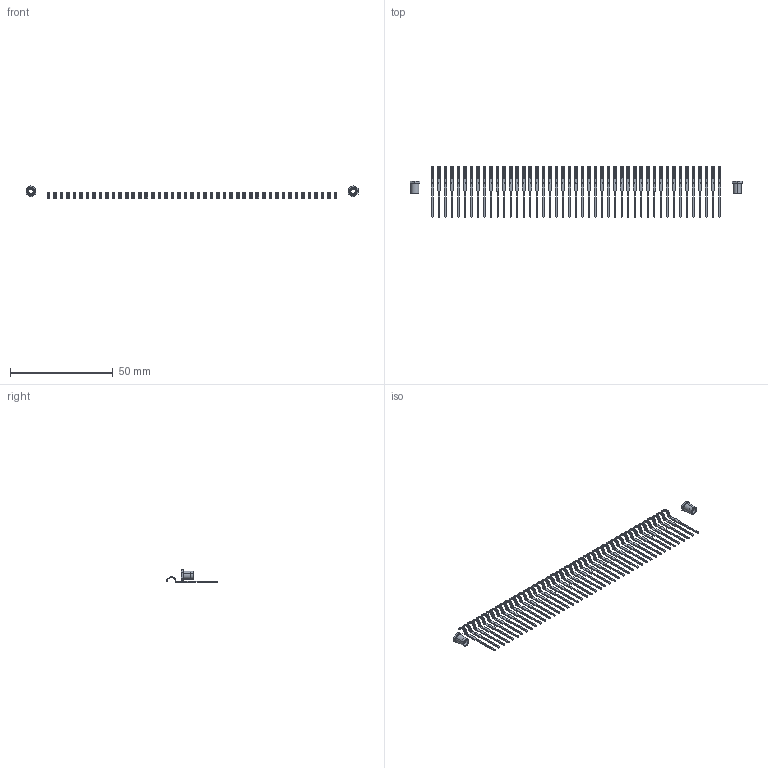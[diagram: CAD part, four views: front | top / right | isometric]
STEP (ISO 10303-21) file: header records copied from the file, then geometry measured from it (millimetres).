
FILE_DESCRIPTION (( 'STEP AP203' ), '1' );
FILE_NAME ('346-045-522-108.STEP', '2018-08-25T03:36:34', ( '' ), ( '' ), 'SwSTEP 2.0', 'SolidWorks 2016', '' );
FILE_SCHEMA (( 'CONFIG_CONTROL_DESIGN' ));
Length unit declared in the file: inch
Products named in the file (4): 345-250-001_345-250-003-102; 346-045-522-108; 346 Part_Flush Mounting Lugs - 0.156 Dia-TI; 345-292-001_345-293-122
Assembly tree (48 placements, depth 2):
  346-045-522-108
    346 Part_Flush Mounting Lugs - 0.156 Dia-TI
    345-292-001_345-293-122  x45
    345-250-001_345-250-003-102  x2
Bounding box: 161.47 x 24.51 x 6.23 mm (x, y, z)
Volume: 619.6 mm3; surface area: 3893.8 mm2
Topology: 47 solids, 47 shells, 2116 faces, 6130 edges, 4020 vertices
Faces by surface type: plane 1368, cylinder 732, cone 12, torus 4
Entity records: 28728 total; most frequent: CARTESIAN_POINT 4906, ORIENTED_EDGE 4878, DIRECTION 4351, EDGE_CURVE 2439, LINE 2107, VECTOR 2107, VERTEX_POINT 1620, AXIS2_PLACEMENT_3D 1122
